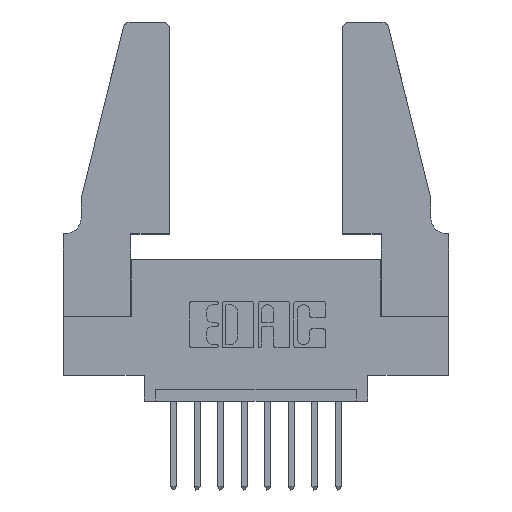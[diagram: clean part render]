
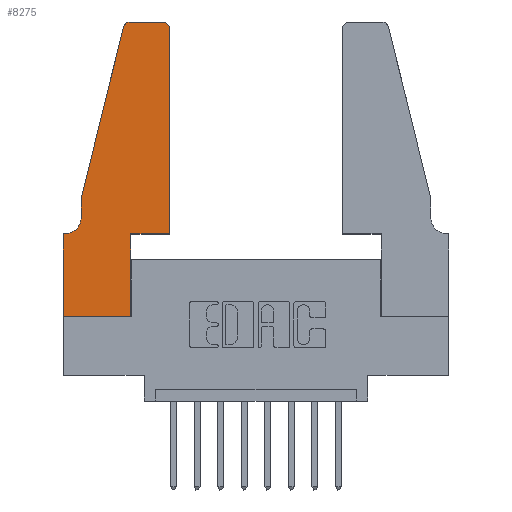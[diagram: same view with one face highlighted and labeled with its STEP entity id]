
A CAD part, top view. The second image highlights one B-rep face of the part: STEP entity #8275.
In plain terms, the highlighted planar face has unit normal (0, 0, 1).
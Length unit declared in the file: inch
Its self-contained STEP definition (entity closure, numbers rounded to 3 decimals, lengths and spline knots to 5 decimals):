
#249 = AXIS2_PLACEMENT_3D ( 'NONE', #11568, #3762, #852 ) ;
#386 = CARTESIAN_POINT ( 'NONE',  ( 0.4205, 1.25, 0.37 ) ) ;
#470 = VECTOR ( 'NONE', #11609, 39.37008 ) ;
#600 = CARTESIAN_POINT ( 'NONE',  ( 0.4505, 0.35, 0.37 ) ) ;
#633 = CARTESIAN_POINT ( 'NONE',  ( 0.25487, 1.22718, 0.37 ) ) ;
#745 = CARTESIAN_POINT ( 'NONE',  ( 0.284, 1.25, 0.37 ) ) ;
#852 = DIRECTION ( 'NONE',  ( -1., 0., 0. ) ) ;
#866 = EDGE_CURVE ( 'NONE', #5618, #3290, #7235, .T. ) ;
#909 = VERTEX_POINT ( 'NONE', #745 ) ;
#972 = AXIS2_PLACEMENT_3D ( 'NONE', #2470, #10391, #4452 ) ;
#1132 = LINE ( 'NONE', #6980, #7379 ) ;
#1203 = DIRECTION ( 'NONE',  ( -1., 0., 0. ) ) ;
#1379 = EDGE_CURVE ( 'NONE', #8096, #1976, #12402, .T. ) ;
#1486 = CARTESIAN_POINT ( 'NONE',  ( 0.4205, 1.22, 0.37 ) ) ;
#1618 = CARTESIAN_POINT ( 'NONE',  ( 0.4505, 0.35, 0.37 ) ) ;
#1976 = VERTEX_POINT ( 'NONE', #6848 ) ;
#2079 = VECTOR ( 'NONE', #5015, 39.37008 ) ;
#2113 = EDGE_CURVE ( 'NONE', #5971, #8096, #1132, .T. ) ;
#2139 = CARTESIAN_POINT ( 'NONE',  ( 0.0755, 0.42, 0.37 ) ) ;
#2198 = LINE ( 'NONE', #3020, #7044 ) ;
#2266 = VERTEX_POINT ( 'NONE', #7227 ) ;
#2470 = CARTESIAN_POINT ( 'NONE',  ( 0., 0.35, 0.37 ) ) ;
#2822 = FACE_OUTER_BOUND ( 'NONE', #6581, .T. ) ;
#3020 = CARTESIAN_POINT ( 'NONE',  ( 0.0755, 0.5, 0.37 ) ) ;
#3075 = CARTESIAN_POINT ( 'NONE',  ( 0.0755, 0.5, 0.37 ) ) ;
#3083 = CIRCLE ( 'NONE', #12414, 0.03 ) ;
#3290 = VERTEX_POINT ( 'NONE', #8866 ) ;
#3511 = DIRECTION ( 'NONE',  ( 1., 0., 0. ) ) ;
#3762 = DIRECTION ( 'NONE',  ( 0., 0., -1. ) ) ;
#3793 = EDGE_CURVE ( 'NONE', #5169, #5618, #11394, .T. ) ;
#3965 = EDGE_CURVE ( 'NONE', #1976, #6093, #3083, .T. ) ;
#4110 = ORIENTED_EDGE ( 'NONE', *, *, #1379, .T. ) ;
#4132 = EDGE_CURVE ( 'NONE', #7665, #2266, #8125, .T. ) ;
#4351 = DIRECTION ( 'NONE',  ( 1., 0., 0. ) ) ;
#4452 = DIRECTION ( 'NONE',  ( 1., 0., 0. ) ) ;
#5015 = DIRECTION ( 'NONE',  ( 1., 0., 0. ) ) ;
#5048 = EDGE_CURVE ( 'NONE', #6093, #909, #12809, .T. ) ;
#5169 = VERTEX_POINT ( 'NONE', #3075 ) ;
#5260 = CARTESIAN_POINT ( 'NONE',  ( 0.2865, 0., 0.37 ) ) ;
#5271 = CIRCLE ( 'NONE', #9877, 0.03 ) ;
#5344 = ORIENTED_EDGE ( 'NONE', *, *, #9232, .T. ) ;
#5618 = VERTEX_POINT ( 'NONE', #2139 ) ;
#5694 = LINE ( 'NONE', #6972, #2079 ) ;
#5706 = VECTOR ( 'NONE', #10696, 39.37008 ) ;
#5971 = VERTEX_POINT ( 'NONE', #7510 ) ;
#6093 = VERTEX_POINT ( 'NONE', #386 ) ;
#6123 = DIRECTION ( 'NONE',  ( 1., 0., 0. ) ) ;
#6168 = VECTOR ( 'NONE', #6565, 39.37008 ) ;
#6272 = CARTESIAN_POINT ( 'NONE',  ( 0.0755, 0.35, 0.37 ) ) ;
#6302 = ORIENTED_EDGE ( 'NONE', *, *, #11689, .T. ) ;
#6404 = DIRECTION ( 'NONE',  ( 0., 0., 1. ) ) ;
#6466 = EDGE_CURVE ( 'NONE', #909, #8850, #5271, .T. ) ;
#6565 = DIRECTION ( 'NONE',  ( 0., 1., 0. ) ) ;
#6581 = EDGE_LOOP ( 'NONE', ( #8935, #8492, #5344, #11953, #12304, #6302, #8788, #9337, #8453, #12882, #4110, #12748 ) ) ;
#6848 = CARTESIAN_POINT ( 'NONE',  ( 0.4505, 1.22, 0.37 ) ) ;
#6972 = CARTESIAN_POINT ( 'NONE',  ( 0., 0., 0.37 ) ) ;
#6980 = CARTESIAN_POINT ( 'NONE',  ( 0.4505, 0.35, 0.37 ) ) ;
#7044 = VECTOR ( 'NONE', #8063, 39.37008 ) ;
#7081 = LINE ( 'NONE', #12531, #6168 ) ;
#7227 = CARTESIAN_POINT ( 'NONE',  ( 0., 0., 0.37 ) ) ;
#7231 = EDGE_CURVE ( 'NONE', #12437, #5971, #7081, .T. ) ;
#7235 = CIRCLE ( 'NONE', #249, 0.07 ) ;
#7379 = VECTOR ( 'NONE', #6123, 39.37008 ) ;
#7510 = CARTESIAN_POINT ( 'NONE',  ( 0.2865, 0.35, 0.37 ) ) ;
#7665 = VERTEX_POINT ( 'NONE', #11871 ) ;
#7677 = EDGE_CURVE ( 'NONE', #2266, #12437, #5694, .T. ) ;
#8010 = DIRECTION ( 'NONE',  ( 0., -1., 0. ) ) ;
#8063 = DIRECTION ( 'NONE',  ( -0.239, -0.971, 0. ) ) ;
#8096 = VERTEX_POINT ( 'NONE', #600 ) ;
#8125 = LINE ( 'NONE', #9550, #470 ) ;
#8275 = ADVANCED_FACE ( 'NONE', ( #2822 ), #9521, .T. ) ;
#8453 = ORIENTED_EDGE ( 'NONE', *, *, #7231, .T. ) ;
#8492 = ORIENTED_EDGE ( 'NONE', *, *, #6466, .T. ) ;
#8549 = CARTESIAN_POINT ( 'NONE',  ( 0.284, 1.22, 0.37 ) ) ;
#8788 = ORIENTED_EDGE ( 'NONE', *, *, #4132, .T. ) ;
#8850 = VERTEX_POINT ( 'NONE', #633 ) ;
#8866 = CARTESIAN_POINT ( 'NONE',  ( 0.0055, 0.35, 0.37 ) ) ;
#8935 = ORIENTED_EDGE ( 'NONE', *, *, #5048, .T. ) ;
#9232 = EDGE_CURVE ( 'NONE', #8850, #5169, #2198, .T. ) ;
#9337 = ORIENTED_EDGE ( 'NONE', *, *, #7677, .T. ) ;
#9494 = VECTOR ( 'NONE', #1203, 39.37008 ) ;
#9521 = PLANE ( 'NONE',  #972 ) ;
#9550 = CARTESIAN_POINT ( 'NONE',  ( 0., 0., 0.37 ) ) ;
#9877 = AXIS2_PLACEMENT_3D ( 'NONE', #8549, #11393, #4351 ) ;
#10391 = DIRECTION ( 'NONE',  ( 0., 0., 1. ) ) ;
#10696 = DIRECTION ( 'NONE',  ( 0., 1., 0. ) ) ;
#10744 = CARTESIAN_POINT ( 'NONE',  ( 0.2605, 1.25, 0.37 ) ) ;
#11106 = VECTOR ( 'NONE', #12805, 39.37008 ) ;
#11393 = DIRECTION ( 'NONE',  ( 0., 0., 1. ) ) ;
#11394 = LINE ( 'NONE', #12021, #11704 ) ;
#11568 = CARTESIAN_POINT ( 'NONE',  ( 0.0055, 0.42, 0.37 ) ) ;
#11609 = DIRECTION ( 'NONE',  ( 0., -1., 0. ) ) ;
#11689 = EDGE_CURVE ( 'NONE', #3290, #7665, #11982, .T. ) ;
#11704 = VECTOR ( 'NONE', #8010, 39.37008 ) ;
#11871 = CARTESIAN_POINT ( 'NONE',  ( 0., 0.35, 0.37 ) ) ;
#11953 = ORIENTED_EDGE ( 'NONE', *, *, #3793, .T. ) ;
#11982 = LINE ( 'NONE', #6272, #9494 ) ;
#12021 = CARTESIAN_POINT ( 'NONE',  ( 0.0755, 0.5, 0.37 ) ) ;
#12304 = ORIENTED_EDGE ( 'NONE', *, *, #866, .T. ) ;
#12402 = LINE ( 'NONE', #1618, #5706 ) ;
#12414 = AXIS2_PLACEMENT_3D ( 'NONE', #1486, #6404, #3511 ) ;
#12437 = VERTEX_POINT ( 'NONE', #5260 ) ;
#12531 = CARTESIAN_POINT ( 'NONE',  ( 0.2865, 0.35, 0.37 ) ) ;
#12748 = ORIENTED_EDGE ( 'NONE', *, *, #3965, .T. ) ;
#12805 = DIRECTION ( 'NONE',  ( -1., 0., 0. ) ) ;
#12809 = LINE ( 'NONE', #10744, #11106 ) ;
#12882 = ORIENTED_EDGE ( 'NONE', *, *, #2113, .T. ) ;
